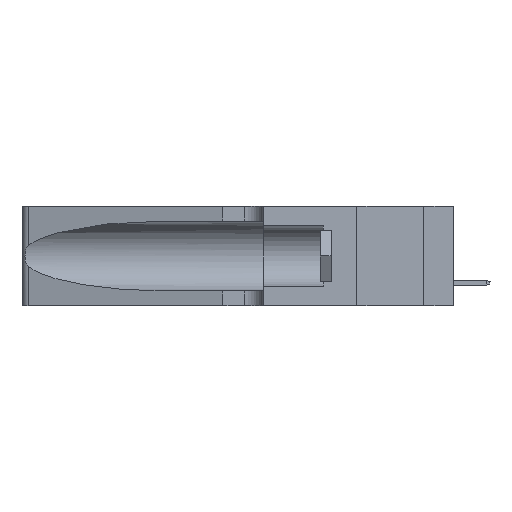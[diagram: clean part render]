
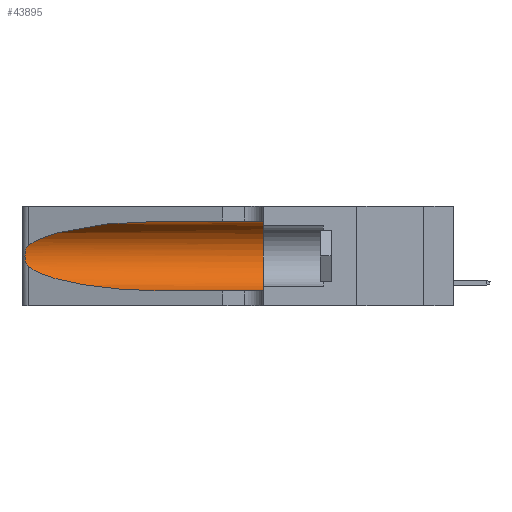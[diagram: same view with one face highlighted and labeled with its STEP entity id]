
A CAD part, left-side view. The second image highlights one B-rep face of the part: STEP entity #43895.
In plain terms, the highlighted cylindrical face has radius 3.308 mm (diameter 6.617 mm), a partial arc.
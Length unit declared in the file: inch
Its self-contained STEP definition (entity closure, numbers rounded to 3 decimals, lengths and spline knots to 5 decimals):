
#1165 = CARTESIAN_POINT ( 'NONE',  ( 0.1305, 0.72297, 0.05475 ) ) ;
#1265 = ORIENTED_EDGE ( 'NONE', *, *, #33429, .T. ) ;
#1876 = CIRCLE ( 'NONE', #47978, 0.13025 ) ;
#2541 = CARTESIAN_POINT ( 'NONE',  ( 0.25487, 1.22718, 0.14631 ) ) ;
#3061 = CARTESIAN_POINT ( 'NONE',  ( 0.26075, 1.23896, 0.178 ) ) ;
#3250 = EDGE_CURVE ( 'NONE', #43117, #27122, #7389, .T. ) ;
#3323 = CARTESIAN_POINT ( 'NONE',  ( 0.1305, 0.35, 0.05475 ) ) ;
#3543 = CARTESIAN_POINT ( 'NONE',  ( 0.1305, 1.61858, 0.31525 ) ) ;
#5219 = ORIENTED_EDGE ( 'NONE', *, *, #43519, .T. ) ;
#5964 = CARTESIAN_POINT ( 'NONE',  ( 0.25555, 1.22994, 0.2215 ) ) ;
#7033 = ORIENTED_EDGE ( 'NONE', *, *, #25639, .F. ) ;
#7389 =( BOUNDED_CURVE ( )  B_SPLINE_CURVE ( 3, ( #36083, #19813, #40281, #31634 ),
 .UNSPECIFIED., .F., .F. ) 
 B_SPLINE_CURVE_WITH_KNOTS ( ( 4, 4 ),
 ( 3.44316, 4.71239 ),
 .UNSPECIFIED. ) 
 CURVE ( )  GEOMETRIC_REPRESENTATION_ITEM ( )  RATIONAL_B_SPLINE_CURVE ( ( 1., 0.87, 0.87, 1. ) ) 
 REPRESENTATION_ITEM ( '' )  );
#8254 = LINE ( 'NONE', #3543, #19504 ) ;
#9663 = CARTESIAN_POINT ( 'NONE',  ( 0.25487, 1.22718, 0.22369 ) ) ;
#10066 = LINE ( 'NONE', #29515, #32602 ) ;
#11978 = FACE_OUTER_BOUND ( 'NONE', #30698, .T. ) ;
#12733 = CARTESIAN_POINT ( 'NONE',  ( 0.1305, 0.72297, 0.31525 ) ) ;
#13790 = CARTESIAN_POINT ( 'NONE',  ( 0.2373, 1.15595, 0.28018 ) ) ;
#13819 = CARTESIAN_POINT ( 'NONE',  ( 0.25487, 1.22718, 0.14631 ) ) ;
#14889 = CARTESIAN_POINT ( 'NONE',  ( 0.25789, 1.23486, 0.15765 ) ) ;
#14948 = DIRECTION ( 'NONE',  ( 0., 0., -1. ) ) ;
#15374 = DIRECTION ( 'NONE',  ( 0., -1., 0. ) ) ;
#15759 = VERTEX_POINT ( 'NONE', #44106 ) ;
#16760 = ORIENTED_EDGE ( 'NONE', *, *, #3250, .T. ) ;
#19089 = CARTESIAN_POINT ( 'NONE',  ( 0.26018, 1.23835, 0.19895 ) ) ;
#19345 = CARTESIAN_POINT ( 'NONE',  ( 0.25854, 1.2359, 0.20912 ) ) ;
#19504 = VECTOR ( 'NONE', #15374, 39.37008 ) ;
#19813 = CARTESIAN_POINT ( 'NONE',  ( 0.2373, 1.15595, 0.08982 ) ) ;
#22004 = CARTESIAN_POINT ( 'NONE',  ( 0.25639, 1.23184, 0.21858 ) ) ;
#22293 = B_SPLINE_CURVE_WITH_KNOTS ( 'NONE', 3,
 ( #9663, #5964, #22004, #47178, #19345, #19089, #47433, #3061, #39296, #35366, #14889, #23548, #38777, #2541 ),
 .UNSPECIFIED., .F., .F.,
 ( 4, 2, 2, 2, 2, 2, 4 ),
 ( 0., 0.00027, 0.00053, 0.00107, 0.0016, 0.00187, 0.00214 ),
 .UNSPECIFIED. ) ;
#23548 = CARTESIAN_POINT ( 'NONE',  ( 0.25639, 1.23186, 0.15144 ) ) ;
#25639 = EDGE_CURVE ( 'NONE', #15759, #49540, #8254, .T. ) ;
#27122 = VERTEX_POINT ( 'NONE', #1165 ) ;
#27295 = EDGE_CURVE ( 'NONE', #49540, #38596, #1876, .T. ) ;
#28754 = CARTESIAN_POINT ( 'NONE',  ( 0.18966, 0.96281, 0.31525 ) ) ;
#29183 = ORIENTED_EDGE ( 'NONE', *, *, #41455, .T. ) ;
#29515 = CARTESIAN_POINT ( 'NONE',  ( 0.1305, 1.61858, 0.05475 ) ) ;
#30142 = AXIS2_PLACEMENT_3D ( 'NONE', #42789, #39815, #14948 ) ;
#30698 = EDGE_LOOP ( 'NONE', ( #1265, #29183, #16760, #5219, #41024, #7033 ) ) ;
#31634 = CARTESIAN_POINT ( 'NONE',  ( 0.1305, 0.72297, 0.05475 ) ) ;
#32602 = VECTOR ( 'NONE', #41589, 39.37008 ) ;
#33429 = EDGE_CURVE ( 'NONE', #15759, #44004, #37923, .T. ) ;
#33748 = DIRECTION ( 'NONE',  ( 0., 1., 0. ) ) ;
#35366 = CARTESIAN_POINT ( 'NONE',  ( 0.25856, 1.23593, 0.16098 ) ) ;
#36083 = CARTESIAN_POINT ( 'NONE',  ( 0.25487, 1.22718, 0.14631 ) ) ;
#37923 =( BOUNDED_CURVE ( )  B_SPLINE_CURVE ( 3, ( #12733, #28754, #13790, #41358 ),
 .UNSPECIFIED., .F., .T. ) 
 B_SPLINE_CURVE_WITH_KNOTS ( ( 4, 4 ),
 ( 1.5708, 2.84003 ),
 .UNSPECIFIED. ) 
 CURVE ( )  GEOMETRIC_REPRESENTATION_ITEM ( )  RATIONAL_B_SPLINE_CURVE ( ( 1., 0.87, 0.87, 1. ) ) 
 REPRESENTATION_ITEM ( '' )  );
#38596 = VERTEX_POINT ( 'NONE', #3323 ) ;
#38777 = CARTESIAN_POINT ( 'NONE',  ( 0.25555, 1.22993, 0.14849 ) ) ;
#39296 = CARTESIAN_POINT ( 'NONE',  ( 0.26017, 1.23833, 0.17102 ) ) ;
#39806 = CARTESIAN_POINT ( 'NONE',  ( 0.1305, 0.35, 0.31525 ) ) ;
#39815 = DIRECTION ( 'NONE',  ( 0., -1., 0. ) ) ;
#40281 = CARTESIAN_POINT ( 'NONE',  ( 0.18966, 0.96281, 0.05475 ) ) ;
#41024 = ORIENTED_EDGE ( 'NONE', *, *, #27295, .F. ) ;
#41358 = CARTESIAN_POINT ( 'NONE',  ( 0.25487, 1.22718, 0.22369 ) ) ;
#41455 = EDGE_CURVE ( 'NONE', #44004, #43117, #22293, .T. ) ;
#41589 = DIRECTION ( 'NONE',  ( 0., -1., 0. ) ) ;
#42789 = CARTESIAN_POINT ( 'NONE',  ( 0.1305, 1.61858, 0.185 ) ) ;
#43117 = VERTEX_POINT ( 'NONE', #13819 ) ;
#43519 = EDGE_CURVE ( 'NONE', #27122, #38596, #10066, .T. ) ;
#43895 = ADVANCED_FACE ( 'NONE', ( #11978 ), #47686, .F. ) ;
#44004 = VERTEX_POINT ( 'NONE', #46728 ) ;
#44106 = CARTESIAN_POINT ( 'NONE',  ( 0.1305, 0.72297, 0.31525 ) ) ;
#46332 = DIRECTION ( 'NONE',  ( 0., 0., 1. ) ) ;
#46728 = CARTESIAN_POINT ( 'NONE',  ( 0.25487, 1.22718, 0.22369 ) ) ;
#47178 = CARTESIAN_POINT ( 'NONE',  ( 0.25787, 1.23484, 0.2124 ) ) ;
#47433 = CARTESIAN_POINT ( 'NONE',  ( 0.26075, 1.23896, 0.19203 ) ) ;
#47686 = CYLINDRICAL_SURFACE ( 'NONE', #30142, 0.13025 ) ;
#47978 = AXIS2_PLACEMENT_3D ( 'NONE', #50785, #33748, #46332 ) ;
#49540 = VERTEX_POINT ( 'NONE', #39806 ) ;
#50785 = CARTESIAN_POINT ( 'NONE',  ( 0.1305, 0.35, 0.185 ) ) ;
